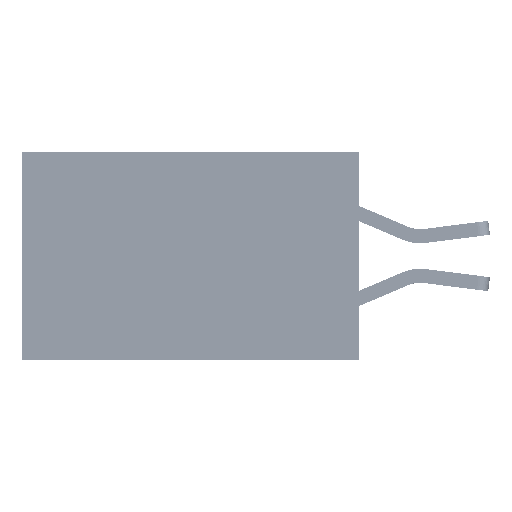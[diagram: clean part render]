
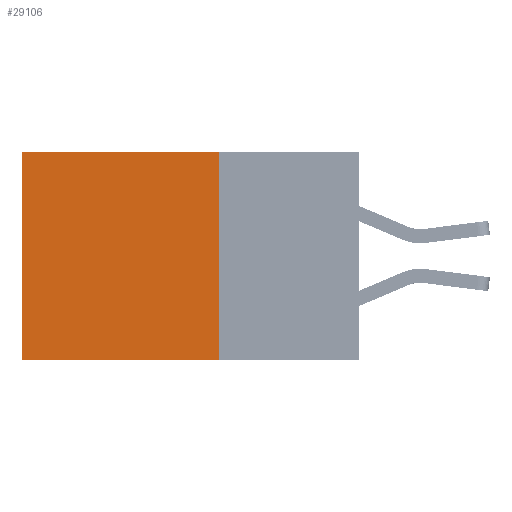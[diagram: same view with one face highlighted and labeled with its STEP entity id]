
A CAD part, left-side view. The second image highlights one B-rep face of the part: STEP entity #29106.
In plain terms, the highlighted planar face has unit normal (-1, 0, 0).
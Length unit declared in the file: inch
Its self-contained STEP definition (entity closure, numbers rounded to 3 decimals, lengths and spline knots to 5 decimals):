
#5522 = CARTESIAN_POINT ( 'NONE',  ( 0.2875, 0.25, 0. ) ) ;
#7327 = VERTEX_POINT ( 'NONE', #28254 ) ;
#7408 = PLANE ( 'NONE',  #27297 ) ;
#8569 = VERTEX_POINT ( 'NONE', #24106 ) ;
#12084 = LINE ( 'NONE', #18389, #26785 ) ;
#13216 = EDGE_CURVE ( 'NONE', #8569, #7327, #17602, .T. ) ;
#15644 = LINE ( 'NONE', #28074, #24411 ) ;
#17602 = LINE ( 'NONE', #23934, #19535 ) ;
#18389 = CARTESIAN_POINT ( 'NONE',  ( 0.2875, 0.25, 0. ) ) ;
#18543 = EDGE_CURVE ( 'NONE', #36448, #8569, #12084, .T. ) ;
#18584 = DIRECTION ( 'NONE',  ( 0., 1., 0. ) ) ;
#19086 = ORIENTED_EDGE ( 'NONE', *, *, #13216, .T. ) ;
#19535 = VECTOR ( 'NONE', #33297, 39.37008 ) ;
#19815 = DIRECTION ( 'NONE',  ( 0., 0., -1. ) ) ;
#23755 = ORIENTED_EDGE ( 'NONE', *, *, #40186, .F. ) ;
#23934 = CARTESIAN_POINT ( 'NONE',  ( 0.2875, 0.6, 0. ) ) ;
#24106 = CARTESIAN_POINT ( 'NONE',  ( 0.2875, 0.6, 0. ) ) ;
#24411 = VECTOR ( 'NONE', #31333, 39.37008 ) ;
#25930 = ORIENTED_EDGE ( 'NONE', *, *, #18543, .T. ) ;
#25938 = FACE_OUTER_BOUND ( 'NONE', #28109, .T. ) ;
#26785 = VECTOR ( 'NONE', #18584, 39.37008 ) ;
#27218 = CARTESIAN_POINT ( 'NONE',  ( 0.2875, 0.25, 0. ) ) ;
#27297 = AXIS2_PLACEMENT_3D ( 'NONE', #38583, #35917, #19815 ) ;
#27478 = VERTEX_POINT ( 'NONE', #40034 ) ;
#27528 = DIRECTION ( 'NONE',  ( 0., 0., -1. ) ) ;
#28074 = CARTESIAN_POINT ( 'NONE',  ( 0.2875, 0.25, -0.37 ) ) ;
#28109 = EDGE_LOOP ( 'NONE', ( #19086, #38729, #23755, #25930 ) ) ;
#28254 = CARTESIAN_POINT ( 'NONE',  ( 0.2875, 0.6, -0.37 ) ) ;
#29106 = ADVANCED_FACE ( 'NONE', ( #25938 ), #7408, .F. ) ;
#31333 = DIRECTION ( 'NONE',  ( 0., 1., 0. ) ) ;
#33297 = DIRECTION ( 'NONE',  ( 0., 0., -1. ) ) ;
#35917 = DIRECTION ( 'NONE',  ( 1., 0., 0. ) ) ;
#36095 = VECTOR ( 'NONE', #27528, 39.37008 ) ;
#36448 = VERTEX_POINT ( 'NONE', #27218 ) ;
#38583 = CARTESIAN_POINT ( 'NONE',  ( 0.2875, 0.25, 0. ) ) ;
#38729 = ORIENTED_EDGE ( 'NONE', *, *, #38874, .F. ) ;
#38874 = EDGE_CURVE ( 'NONE', #27478, #7327, #15644, .T. ) ;
#39559 = LINE ( 'NONE', #5522, #36095 ) ;
#40034 = CARTESIAN_POINT ( 'NONE',  ( 0.2875, 0.25, -0.37 ) ) ;
#40186 = EDGE_CURVE ( 'NONE', #36448, #27478, #39559, .T. ) ;
